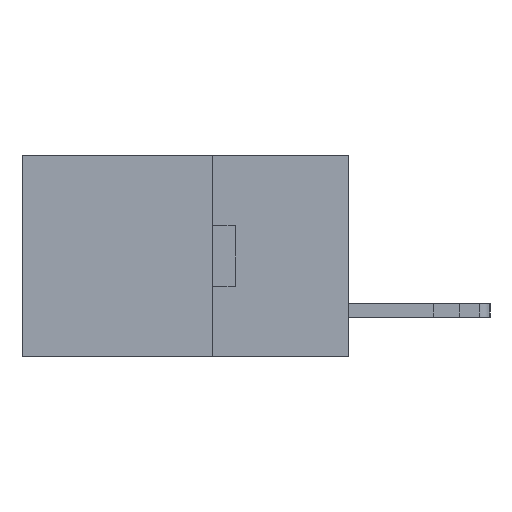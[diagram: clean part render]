
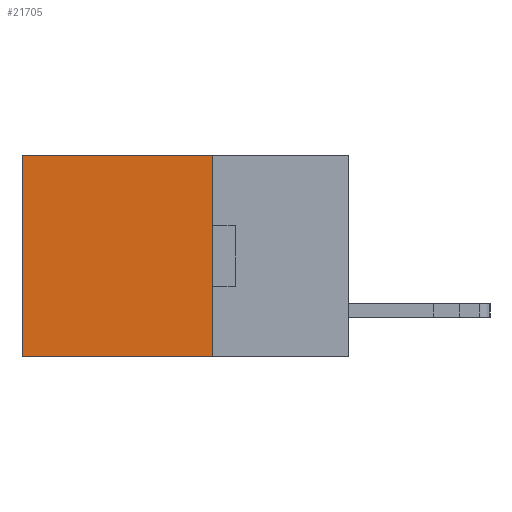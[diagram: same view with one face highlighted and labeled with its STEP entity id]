
A CAD part, left-side view. The second image highlights one B-rep face of the part: STEP entity #21705.
In plain terms, the highlighted planar face has unit normal (-1, 0, 0).
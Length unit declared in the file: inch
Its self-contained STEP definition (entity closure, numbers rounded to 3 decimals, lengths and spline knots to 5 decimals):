
#712 = DIRECTION ( 'NONE',  ( 0., 0., -1. ) ) ;
#2163 = DIRECTION ( 'NONE',  ( 0., 1., 0. ) ) ;
#2825 = CARTESIAN_POINT ( 'NONE',  ( 0.2615, 0.25, -0.37 ) ) ;
#4786 = LINE ( 'NONE', #13530, #20823 ) ;
#6984 = LINE ( 'NONE', #12705, #17499 ) ;
#7120 = EDGE_LOOP ( 'NONE', ( #19143, #26470, #8867, #22303 ) ) ;
#8714 = VECTOR ( 'NONE', #16114, 39.37008 ) ;
#8867 = ORIENTED_EDGE ( 'NONE', *, *, #9236, .F. ) ;
#9092 = CARTESIAN_POINT ( 'NONE',  ( 0.2615, 0.25, -0.37 ) ) ;
#9236 = EDGE_CURVE ( 'NONE', #23692, #12159, #12674, .T. ) ;
#9542 = EDGE_CURVE ( 'NONE', #23692, #10446, #4786, .T. ) ;
#10446 = VERTEX_POINT ( 'NONE', #15915 ) ;
#10590 = DIRECTION ( 'NONE',  ( 0., 0., -1. ) ) ;
#11324 = PLANE ( 'NONE',  #14548 ) ;
#12159 = VERTEX_POINT ( 'NONE', #9092 ) ;
#12674 = LINE ( 'NONE', #21006, #17585 ) ;
#12705 = CARTESIAN_POINT ( 'NONE',  ( 0.2615, 0.25, -0.37 ) ) ;
#12723 = CARTESIAN_POINT ( 'NONE',  ( 0.2615, 0.6, -0.37 ) ) ;
#13446 = DIRECTION ( 'NONE',  ( 1., 0., 0. ) ) ;
#13530 = CARTESIAN_POINT ( 'NONE',  ( 0.2615, 0.25, 0. ) ) ;
#14548 = AXIS2_PLACEMENT_3D ( 'NONE', #2825, #13446, #712 ) ;
#15595 = DIRECTION ( 'NONE',  ( 0., 1., 0. ) ) ;
#15915 = CARTESIAN_POINT ( 'NONE',  ( 0.2615, 0.6, 0. ) ) ;
#16114 = DIRECTION ( 'NONE',  ( 0., 0., -1. ) ) ;
#17499 = VECTOR ( 'NONE', #2163, 39.37008 ) ;
#17585 = VECTOR ( 'NONE', #10590, 39.37008 ) ;
#18167 = VERTEX_POINT ( 'NONE', #12723 ) ;
#19143 = ORIENTED_EDGE ( 'NONE', *, *, #26976, .T. ) ;
#19847 = LINE ( 'NONE', #22403, #8714 ) ;
#20823 = VECTOR ( 'NONE', #15595, 39.37008 ) ;
#21006 = CARTESIAN_POINT ( 'NONE',  ( 0.2615, 0.25, -0.37 ) ) ;
#21505 = EDGE_CURVE ( 'NONE', #12159, #18167, #6984, .T. ) ;
#21705 = ADVANCED_FACE ( 'NONE', ( #22022 ), #11324, .F. ) ;
#22022 = FACE_OUTER_BOUND ( 'NONE', #7120, .T. ) ;
#22303 = ORIENTED_EDGE ( 'NONE', *, *, #9542, .T. ) ;
#22403 = CARTESIAN_POINT ( 'NONE',  ( 0.2615, 0.6, -0.37 ) ) ;
#23692 = VERTEX_POINT ( 'NONE', #24817 ) ;
#24817 = CARTESIAN_POINT ( 'NONE',  ( 0.2615, 0.25, 0. ) ) ;
#26470 = ORIENTED_EDGE ( 'NONE', *, *, #21505, .F. ) ;
#26976 = EDGE_CURVE ( 'NONE', #10446, #18167, #19847, .T. ) ;
